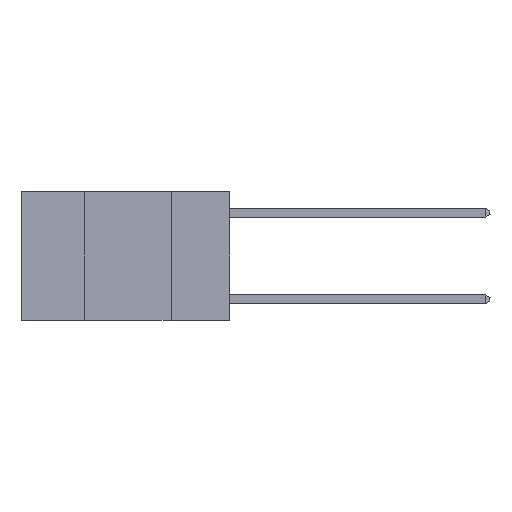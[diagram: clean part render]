
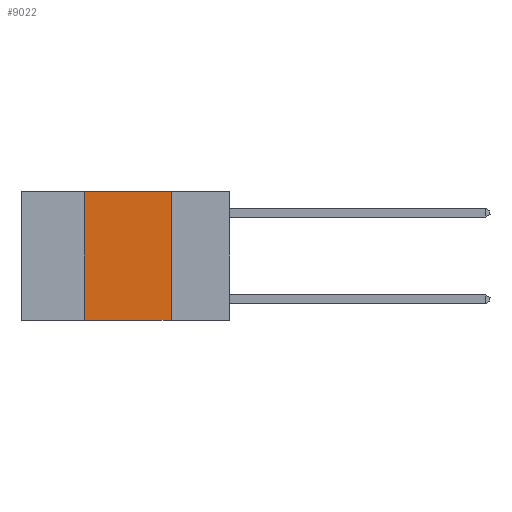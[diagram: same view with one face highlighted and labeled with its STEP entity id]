
A CAD part, left-side view. The second image highlights one B-rep face of the part: STEP entity #9022.
In plain terms, the highlighted planar face has unit normal (-1, 0, 0).
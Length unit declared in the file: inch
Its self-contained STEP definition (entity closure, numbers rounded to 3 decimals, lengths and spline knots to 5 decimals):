
#671 = LINE ( 'NONE', #4485, #10616 ) ;
#2279 = EDGE_CURVE ( 'NONE', #3866, #22187, #10459, .T. ) ;
#2548 = ORIENTED_EDGE ( 'NONE', *, *, #10561, .T. ) ;
#3436 = DIRECTION ( 'NONE',  ( 0., -1., 0. ) ) ;
#3866 = VERTEX_POINT ( 'NONE', #14180 ) ;
#4342 = CARTESIAN_POINT ( 'NONE',  ( 0., 0.17, 0. ) ) ;
#4485 = CARTESIAN_POINT ( 'NONE',  ( 0., 0.17, 0. ) ) ;
#4823 = CARTESIAN_POINT ( 'NONE',  ( 0., 0.6, 0. ) ) ;
#5785 = VERTEX_POINT ( 'NONE', #4342 ) ;
#5809 = DIRECTION ( 'NONE',  ( 0., -1., 0. ) ) ;
#6485 = EDGE_CURVE ( 'NONE', #5785, #20771, #671, .T. ) ;
#6942 = ORIENTED_EDGE ( 'NONE', *, *, #2279, .F. ) ;
#7295 = FACE_OUTER_BOUND ( 'NONE', #13094, .T. ) ;
#7705 = DIRECTION ( 'NONE',  ( 0., 0., -1. ) ) ;
#8620 = CARTESIAN_POINT ( 'NONE',  ( 0., 0.42, 0. ) ) ;
#9022 = ADVANCED_FACE ( 'NONE', ( #7295 ), #14221, .F. ) ;
#9592 = CARTESIAN_POINT ( 'NONE',  ( 0., 0.17, -0.37 ) ) ;
#10399 = CARTESIAN_POINT ( 'NONE',  ( 0., 0.6, 0. ) ) ;
#10459 = LINE ( 'NONE', #8620, #19942 ) ;
#10561 = EDGE_CURVE ( 'NONE', #3866, #20771, #18163, .T. ) ;
#10616 = VECTOR ( 'NONE', #7705, 39.37008 ) ;
#11098 = VECTOR ( 'NONE', #3436, 39.37008 ) ;
#11471 = CARTESIAN_POINT ( 'NONE',  ( 0., 0.42, 0. ) ) ;
#12212 = VECTOR ( 'NONE', #5809, 39.37008 ) ;
#12252 = DIRECTION ( 'NONE',  ( 1., 0., 0. ) ) ;
#13094 = EDGE_LOOP ( 'NONE', ( #21753, #19370, #6942, #2548 ) ) ;
#14180 = CARTESIAN_POINT ( 'NONE',  ( 0., 0.42, -0.37 ) ) ;
#14188 = AXIS2_PLACEMENT_3D ( 'NONE', #10399, #12252, #19440 ) ;
#14221 = PLANE ( 'NONE',  #14188 ) ;
#14791 = CARTESIAN_POINT ( 'NONE',  ( 0., 0.6, -0.37 ) ) ;
#18163 = LINE ( 'NONE', #14791, #12212 ) ;
#19039 = DIRECTION ( 'NONE',  ( 0., 0., 1. ) ) ;
#19140 = LINE ( 'NONE', #4823, #11098 ) ;
#19370 = ORIENTED_EDGE ( 'NONE', *, *, #21837, .F. ) ;
#19440 = DIRECTION ( 'NONE',  ( 0., 0., -1. ) ) ;
#19942 = VECTOR ( 'NONE', #19039, 39.37008 ) ;
#20771 = VERTEX_POINT ( 'NONE', #9592 ) ;
#21753 = ORIENTED_EDGE ( 'NONE', *, *, #6485, .F. ) ;
#21837 = EDGE_CURVE ( 'NONE', #22187, #5785, #19140, .T. ) ;
#22187 = VERTEX_POINT ( 'NONE', #11471 ) ;
